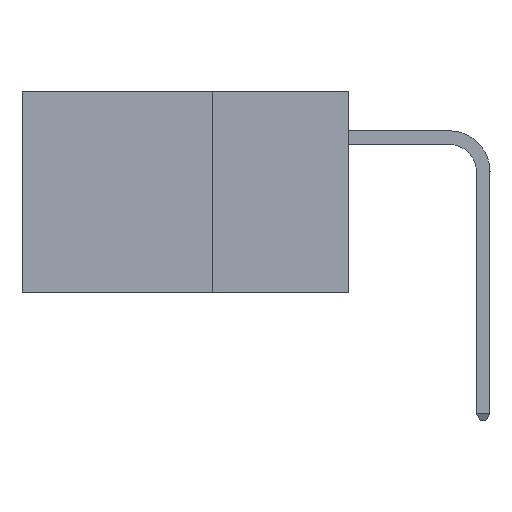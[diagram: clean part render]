
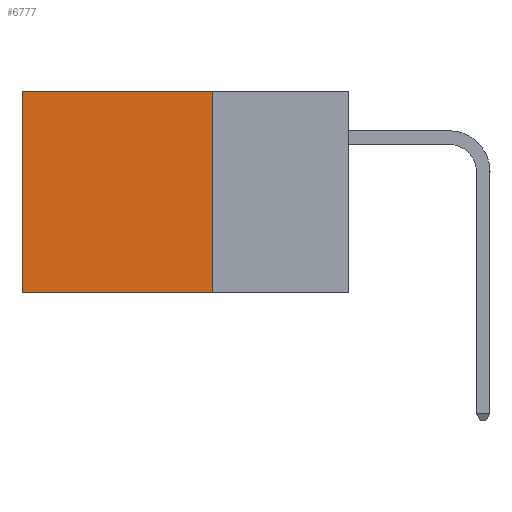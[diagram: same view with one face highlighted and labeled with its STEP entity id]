
A CAD part, left-side view. The second image highlights one B-rep face of the part: STEP entity #6777.
In plain terms, the highlighted planar face has unit normal (-1, 0, 0).
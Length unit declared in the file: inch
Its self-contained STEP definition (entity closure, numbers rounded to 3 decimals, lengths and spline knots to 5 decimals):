
#1000 = CARTESIAN_POINT ( 'NONE',  ( 0.2875, 0.25, 0. ) ) ;
#2774 = EDGE_CURVE ( 'NONE', #10932, #9217, #11730, .T. ) ;
#3029 = DIRECTION ( 'NONE',  ( 0., 1., 0. ) ) ;
#3601 = CARTESIAN_POINT ( 'NONE',  ( 0.2875, 0.25, -0.37 ) ) ;
#4224 = CARTESIAN_POINT ( 'NONE',  ( 0.2875, 0.6, 0. ) ) ;
#5585 = DIRECTION ( 'NONE',  ( 0., 1., 0. ) ) ;
#6052 = VECTOR ( 'NONE', #9276, 39.37008 ) ;
#6607 = LINE ( 'NONE', #3601, #16133 ) ;
#6765 = CARTESIAN_POINT ( 'NONE',  ( 0.2875, 0.25, -0.37 ) ) ;
#6777 = ADVANCED_FACE ( 'NONE', ( #10062 ), #7500, .F. ) ;
#7500 = PLANE ( 'NONE',  #11932 ) ;
#9031 = EDGE_CURVE ( 'NONE', #23599, #20721, #20978, .T. ) ;
#9077 = CARTESIAN_POINT ( 'NONE',  ( 0.2875, 0.6, 0. ) ) ;
#9217 = VERTEX_POINT ( 'NONE', #6765 ) ;
#9276 = DIRECTION ( 'NONE',  ( 0., 0., -1. ) ) ;
#9398 = DIRECTION ( 'NONE',  ( 0., 0., -1. ) ) ;
#9760 = CARTESIAN_POINT ( 'NONE',  ( 0.2875, 0.6, -0.37 ) ) ;
#9886 = ORIENTED_EDGE ( 'NONE', *, *, #21688, .T. ) ;
#10037 = ORIENTED_EDGE ( 'NONE', *, *, #2774, .F. ) ;
#10062 = FACE_OUTER_BOUND ( 'NONE', #21665, .T. ) ;
#10932 = VERTEX_POINT ( 'NONE', #19707 ) ;
#11434 = VECTOR ( 'NONE', #23186, 39.37008 ) ;
#11730 = LINE ( 'NONE', #15026, #6052 ) ;
#11760 = LINE ( 'NONE', #1000, #20718 ) ;
#11885 = ORIENTED_EDGE ( 'NONE', *, *, #9031, .T. ) ;
#11932 = AXIS2_PLACEMENT_3D ( 'NONE', #18899, #20818, #9398 ) ;
#15026 = CARTESIAN_POINT ( 'NONE',  ( 0.2875, 0.25, 0. ) ) ;
#16133 = VECTOR ( 'NONE', #5585, 39.37008 ) ;
#16963 = EDGE_CURVE ( 'NONE', #9217, #20721, #6607, .T. ) ;
#17623 = ORIENTED_EDGE ( 'NONE', *, *, #16963, .F. ) ;
#18899 = CARTESIAN_POINT ( 'NONE',  ( 0.2875, 0.25, 0. ) ) ;
#19707 = CARTESIAN_POINT ( 'NONE',  ( 0.2875, 0.25, 0. ) ) ;
#20718 = VECTOR ( 'NONE', #3029, 39.37008 ) ;
#20721 = VERTEX_POINT ( 'NONE', #9760 ) ;
#20818 = DIRECTION ( 'NONE',  ( 1., 0., 0. ) ) ;
#20978 = LINE ( 'NONE', #4224, #11434 ) ;
#21665 = EDGE_LOOP ( 'NONE', ( #11885, #17623, #10037, #9886 ) ) ;
#21688 = EDGE_CURVE ( 'NONE', #10932, #23599, #11760, .T. ) ;
#23186 = DIRECTION ( 'NONE',  ( 0., 0., -1. ) ) ;
#23599 = VERTEX_POINT ( 'NONE', #9077 ) ;
